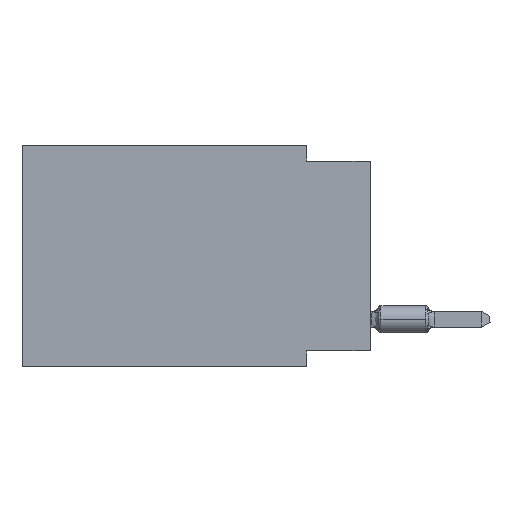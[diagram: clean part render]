
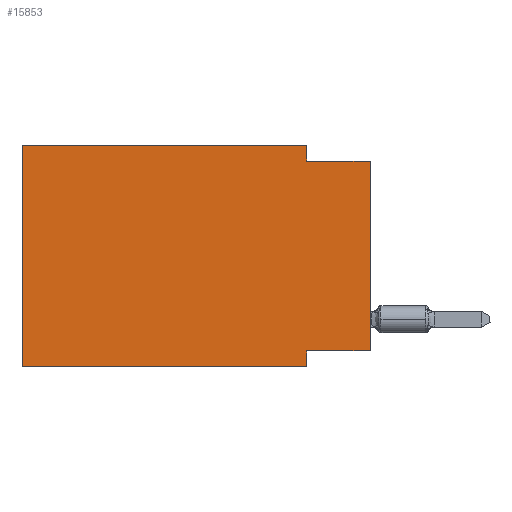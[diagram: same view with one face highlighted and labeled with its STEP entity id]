
A CAD part, left-side view. The second image highlights one B-rep face of the part: STEP entity #15853.
In plain terms, the highlighted planar face has unit normal (-1, 0, 0).
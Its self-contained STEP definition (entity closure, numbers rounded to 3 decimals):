
#710 = CARTESIAN_POINT ( 'NONE',  ( 0., 0., -8.255 ) ) ;
#1826 = DIRECTION ( 'NONE',  ( 0., -1., 0. ) ) ;
#2571 = CARTESIAN_POINT ( 'NONE',  ( 0., 13.97, 0. ) ) ;
#3128 = LINE ( 'NONE', #710, #3766 ) ;
#3207 = EDGE_CURVE ( 'NONE', #13064, #22945, #11157, .T. ) ;
#3225 = VECTOR ( 'NONE', #28816, 1000. ) ;
#3682 = VERTEX_POINT ( 'NONE', #3864 ) ;
#3766 = VECTOR ( 'NONE', #30297, 1000. ) ;
#3864 = CARTESIAN_POINT ( 'NONE',  ( 0., 2.54, -8.255 ) ) ;
#4153 = VECTOR ( 'NONE', #17005, 1000. ) ;
#4790 = ORIENTED_EDGE ( 'NONE', *, *, #10780, .F. ) ;
#4871 = CARTESIAN_POINT ( 'NONE',  ( 0., 13.97, 0. ) ) ;
#5017 = EDGE_CURVE ( 'NONE', #24064, #27546, #19293, .T. ) ;
#5354 = CARTESIAN_POINT ( 'NONE',  ( 0., 0., -0.635 ) ) ;
#5783 = ORIENTED_EDGE ( 'NONE', *, *, #20767, .F. ) ;
#6510 = ORIENTED_EDGE ( 'NONE', *, *, #16418, .F. ) ;
#6646 = DIRECTION ( 'NONE',  ( 0., 0., -1. ) ) ;
#6894 = ORIENTED_EDGE ( 'NONE', *, *, #13358, .F. ) ;
#6973 = LINE ( 'NONE', #21858, #4153 ) ;
#7610 = DIRECTION ( 'NONE',  ( 1., 0., 0. ) ) ;
#8325 = DIRECTION ( 'NONE',  ( 0., 0., -1. ) ) ;
#9233 = EDGE_CURVE ( 'NONE', #9706, #27546, #17200, .T. ) ;
#9706 = VERTEX_POINT ( 'NONE', #23960 ) ;
#10355 = ORIENTED_EDGE ( 'NONE', *, *, #5017, .T. ) ;
#10756 = LINE ( 'NONE', #30468, #11631 ) ;
#10780 = EDGE_CURVE ( 'NONE', #3682, #22945, #11501, .T. ) ;
#11157 = LINE ( 'NONE', #18450, #11977 ) ;
#11501 = LINE ( 'NONE', #21373, #25295 ) ;
#11631 = VECTOR ( 'NONE', #8325, 1000. ) ;
#11977 = VECTOR ( 'NONE', #23941, 1000. ) ;
#12316 = EDGE_CURVE ( 'NONE', #13064, #29692, #6973, .T. ) ;
#13064 = VERTEX_POINT ( 'NONE', #13693 ) ;
#13358 = EDGE_CURVE ( 'NONE', #24064, #3682, #3128, .T. ) ;
#13693 = CARTESIAN_POINT ( 'NONE',  ( 0., 13.97, -8.89 ) ) ;
#15373 = DIRECTION ( 'NONE',  ( 0., 0., -1. ) ) ;
#15724 = VECTOR ( 'NONE', #31861, 1000. ) ;
#15853 = ADVANCED_FACE ( 'NONE', ( #29455 ), #27021, .F. ) ;
#15897 = ORIENTED_EDGE ( 'NONE', *, *, #3207, .T. ) ;
#16418 = EDGE_CURVE ( 'NONE', #27299, #9706, #10756, .T. ) ;
#16808 = CARTESIAN_POINT ( 'NONE',  ( 0., 0., -8.255 ) ) ;
#16975 = CARTESIAN_POINT ( 'NONE',  ( 0., 13.97, 0. ) ) ;
#17005 = DIRECTION ( 'NONE',  ( 0., 0., 1. ) ) ;
#17200 = LINE ( 'NONE', #31591, #26730 ) ;
#17582 = EDGE_LOOP ( 'NONE', ( #10355, #27915, #6510, #5783, #25375, #15897, #4790, #6894 ) ) ;
#18450 = CARTESIAN_POINT ( 'NONE',  ( 0., 13.97, -8.89 ) ) ;
#18965 = CARTESIAN_POINT ( 'NONE',  ( 0., 0., 0. ) ) ;
#19293 = LINE ( 'NONE', #18965, #3225 ) ;
#20767 = EDGE_CURVE ( 'NONE', #29692, #27299, #24281, .T. ) ;
#21373 = CARTESIAN_POINT ( 'NONE',  ( 0., 2.54, -8.89 ) ) ;
#21858 = CARTESIAN_POINT ( 'NONE',  ( 0., 13.97, 0. ) ) ;
#22945 = VERTEX_POINT ( 'NONE', #23760 ) ;
#23760 = CARTESIAN_POINT ( 'NONE',  ( 0., 2.54, -8.89 ) ) ;
#23941 = DIRECTION ( 'NONE',  ( 0., -1., 0. ) ) ;
#23960 = CARTESIAN_POINT ( 'NONE',  ( 0., 2.54, -0.635 ) ) ;
#24064 = VERTEX_POINT ( 'NONE', #16808 ) ;
#24281 = LINE ( 'NONE', #2571, #15724 ) ;
#25295 = VECTOR ( 'NONE', #6646, 1000. ) ;
#25375 = ORIENTED_EDGE ( 'NONE', *, *, #12316, .F. ) ;
#26730 = VECTOR ( 'NONE', #1826, 1000. ) ;
#27021 = PLANE ( 'NONE',  #30235 ) ;
#27299 = VERTEX_POINT ( 'NONE', #27707 ) ;
#27546 = VERTEX_POINT ( 'NONE', #5354 ) ;
#27707 = CARTESIAN_POINT ( 'NONE',  ( 0., 2.54, 0. ) ) ;
#27915 = ORIENTED_EDGE ( 'NONE', *, *, #9233, .F. ) ;
#28816 = DIRECTION ( 'NONE',  ( 0., 0., 1. ) ) ;
#29455 = FACE_OUTER_BOUND ( 'NONE', #17582, .T. ) ;
#29692 = VERTEX_POINT ( 'NONE', #16975 ) ;
#30235 = AXIS2_PLACEMENT_3D ( 'NONE', #4871, #7610, #15373 ) ;
#30297 = DIRECTION ( 'NONE',  ( 0., 1., 0. ) ) ;
#30468 = CARTESIAN_POINT ( 'NONE',  ( 0., 2.54, 0. ) ) ;
#31591 = CARTESIAN_POINT ( 'NONE',  ( 0., 0., -0.635 ) ) ;
#31861 = DIRECTION ( 'NONE',  ( 0., -1., 0. ) ) ;
